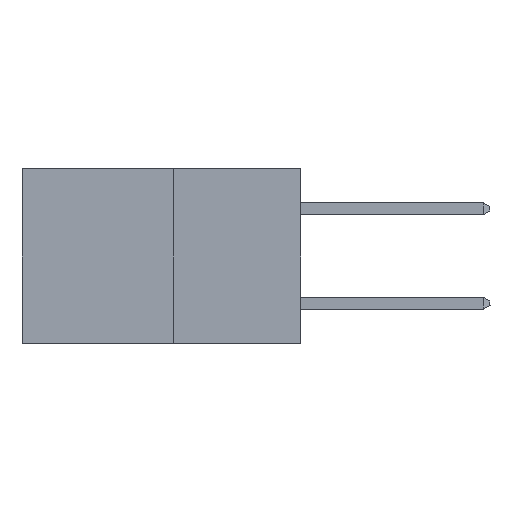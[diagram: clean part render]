
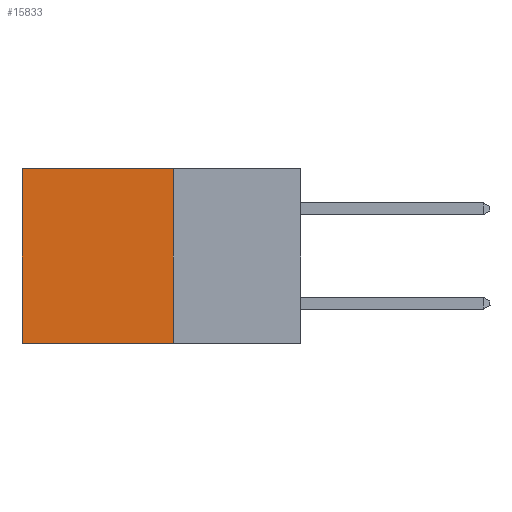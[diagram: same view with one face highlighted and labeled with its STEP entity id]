
A CAD part, left-side view. The second image highlights one B-rep face of the part: STEP entity #15833.
In plain terms, the highlighted planar face has unit normal (-1, 0, 0).
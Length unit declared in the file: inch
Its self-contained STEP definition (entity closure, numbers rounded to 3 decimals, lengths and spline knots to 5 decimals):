
#35 = EDGE_CURVE ( 'NONE', #20091, #656, #15655, .T. ) ;
#79 = DIRECTION ( 'NONE',  ( 0., 0., -1. ) ) ;
#656 = VERTEX_POINT ( 'NONE', #18015 ) ;
#703 = CARTESIAN_POINT ( 'NONE',  ( 0.277, 0.27, 0. ) ) ;
#1323 = FACE_OUTER_BOUND ( 'NONE', #6213, .T. ) ;
#1587 = AXIS2_PLACEMENT_3D ( 'NONE', #8895, #10653, #79 ) ;
#1592 = VECTOR ( 'NONE', #18854, 39.37008 ) ;
#2120 = LINE ( 'NONE', #22687, #20389 ) ;
#2952 = DIRECTION ( 'NONE',  ( 0., 1., 0. ) ) ;
#2987 = ORIENTED_EDGE ( 'NONE', *, *, #8265, .T. ) ;
#3215 = ORIENTED_EDGE ( 'NONE', *, *, #7204, .F. ) ;
#4203 = VERTEX_POINT ( 'NONE', #8200 ) ;
#6205 = VECTOR ( 'NONE', #2952, 39.37008 ) ;
#6213 = EDGE_LOOP ( 'NONE', ( #2987, #8486, #3215, #15288 ) ) ;
#7204 = EDGE_CURVE ( 'NONE', #20091, #4203, #21281, .T. ) ;
#8200 = CARTESIAN_POINT ( 'NONE',  ( 0.277, 0.27, -0.37 ) ) ;
#8245 = CARTESIAN_POINT ( 'NONE',  ( 0.277, 0.59, -0.37 ) ) ;
#8265 = EDGE_CURVE ( 'NONE', #656, #10795, #19868, .T. ) ;
#8486 = ORIENTED_EDGE ( 'NONE', *, *, #17138, .F. ) ;
#8895 = CARTESIAN_POINT ( 'NONE',  ( 0.277, 0.27, -0.37 ) ) ;
#10653 = DIRECTION ( 'NONE',  ( 1., 0., 0. ) ) ;
#10795 = VERTEX_POINT ( 'NONE', #21428 ) ;
#13121 = DIRECTION ( 'NONE',  ( 0., 0., -1. ) ) ;
#13235 = CARTESIAN_POINT ( 'NONE',  ( 0.277, 0.27, -0.37 ) ) ;
#15288 = ORIENTED_EDGE ( 'NONE', *, *, #35, .T. ) ;
#15546 = CARTESIAN_POINT ( 'NONE',  ( 0.277, 0.27, 0. ) ) ;
#15655 = LINE ( 'NONE', #15546, #6205 ) ;
#15833 = ADVANCED_FACE ( 'NONE', ( #1323 ), #19499, .F. ) ;
#16629 = VECTOR ( 'NONE', #13121, 39.37008 ) ;
#17138 = EDGE_CURVE ( 'NONE', #4203, #10795, #2120, .T. ) ;
#18015 = CARTESIAN_POINT ( 'NONE',  ( 0.277, 0.59, 0. ) ) ;
#18854 = DIRECTION ( 'NONE',  ( 0., 0., -1. ) ) ;
#19499 = PLANE ( 'NONE',  #1587 ) ;
#19868 = LINE ( 'NONE', #8245, #1592 ) ;
#20091 = VERTEX_POINT ( 'NONE', #703 ) ;
#20389 = VECTOR ( 'NONE', #21040, 39.37008 ) ;
#21040 = DIRECTION ( 'NONE',  ( 0., 1., 0. ) ) ;
#21281 = LINE ( 'NONE', #13235, #16629 ) ;
#21428 = CARTESIAN_POINT ( 'NONE',  ( 0.277, 0.59, -0.37 ) ) ;
#22687 = CARTESIAN_POINT ( 'NONE',  ( 0.277, 0.27, -0.37 ) ) ;
